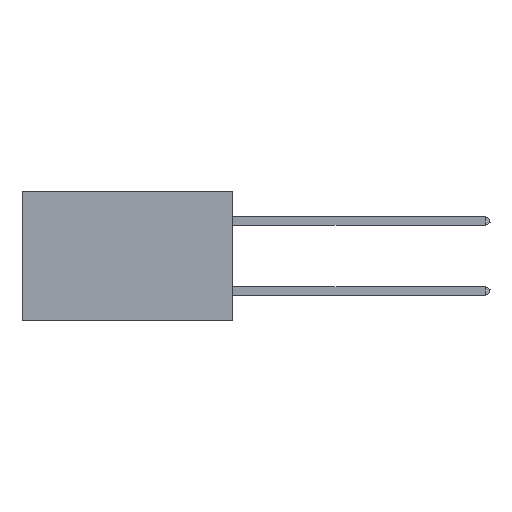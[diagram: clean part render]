
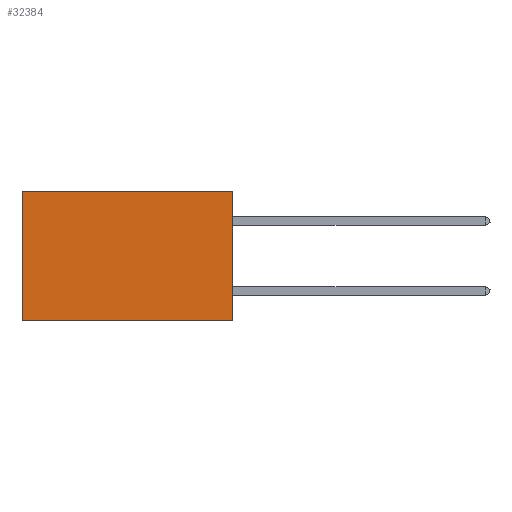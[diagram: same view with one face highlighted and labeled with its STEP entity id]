
A CAD part, left-side view. The second image highlights one B-rep face of the part: STEP entity #32384.
In plain terms, the highlighted planar face has unit normal (-1, 0, 0).
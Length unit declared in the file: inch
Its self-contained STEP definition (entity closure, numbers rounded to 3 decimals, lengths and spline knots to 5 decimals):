
#680 = EDGE_CURVE ( 'NONE', #29139, #26061, #40284, .T. ) ;
#997 = VECTOR ( 'NONE', #4630, 39.37008 ) ;
#1095 = ORIENTED_EDGE ( 'NONE', *, *, #31149, .T. ) ;
#1364 = CARTESIAN_POINT ( 'NONE',  ( 0.2875, 0., 0. ) ) ;
#2033 = DIRECTION ( 'NONE',  ( 0., 0., -1. ) ) ;
#3437 = LINE ( 'NONE', #18632, #30656 ) ;
#4630 = DIRECTION ( 'NONE',  ( 0., 1., 0. ) ) ;
#8059 = CARTESIAN_POINT ( 'NONE',  ( 0.2875, 0., 0. ) ) ;
#8118 = PLANE ( 'NONE',  #23854 ) ;
#8789 = CARTESIAN_POINT ( 'NONE',  ( 0.2875, 0.6, 0. ) ) ;
#10170 = CARTESIAN_POINT ( 'NONE',  ( 0.2875, 0., -0.37 ) ) ;
#10441 = VERTEX_POINT ( 'NONE', #27343 ) ;
#11585 = DIRECTION ( 'NONE',  ( 1., 0., 0. ) ) ;
#14887 = DIRECTION ( 'NONE',  ( 0., 1., 0. ) ) ;
#15821 = LINE ( 'NONE', #35925, #997 ) ;
#17450 = DIRECTION ( 'NONE',  ( 0., 0., -1. ) ) ;
#17477 = VECTOR ( 'NONE', #17450, 39.37008 ) ;
#18632 = CARTESIAN_POINT ( 'NONE',  ( 0.2875, 0.6, 0. ) ) ;
#20825 = CARTESIAN_POINT ( 'NONE',  ( 0.2875, 0., 0. ) ) ;
#23167 = LINE ( 'NONE', #37450, #35593 ) ;
#23475 = EDGE_CURVE ( 'NONE', #28111, #10441, #3437, .T. ) ;
#23854 = AXIS2_PLACEMENT_3D ( 'NONE', #20825, #11585, #2033 ) ;
#25884 = EDGE_LOOP ( 'NONE', ( #33829, #30295, #36092, #1095 ) ) ;
#26061 = VERTEX_POINT ( 'NONE', #10170 ) ;
#27343 = CARTESIAN_POINT ( 'NONE',  ( 0.2875, 0.6, -0.37 ) ) ;
#28111 = VERTEX_POINT ( 'NONE', #8789 ) ;
#29139 = VERTEX_POINT ( 'NONE', #1364 ) ;
#29758 = EDGE_CURVE ( 'NONE', #26061, #10441, #15821, .T. ) ;
#30295 = ORIENTED_EDGE ( 'NONE', *, *, #29758, .F. ) ;
#30656 = VECTOR ( 'NONE', #30829, 39.37008 ) ;
#30829 = DIRECTION ( 'NONE',  ( 0., 0., -1. ) ) ;
#31149 = EDGE_CURVE ( 'NONE', #29139, #28111, #23167, .T. ) ;
#32384 = ADVANCED_FACE ( 'NONE', ( #34502 ), #8118, .F. ) ;
#33829 = ORIENTED_EDGE ( 'NONE', *, *, #23475, .T. ) ;
#34502 = FACE_OUTER_BOUND ( 'NONE', #25884, .T. ) ;
#35593 = VECTOR ( 'NONE', #14887, 39.37008 ) ;
#35925 = CARTESIAN_POINT ( 'NONE',  ( 0.2875, 0., -0.37 ) ) ;
#36092 = ORIENTED_EDGE ( 'NONE', *, *, #680, .F. ) ;
#37450 = CARTESIAN_POINT ( 'NONE',  ( 0.2875, 0., 0. ) ) ;
#40284 = LINE ( 'NONE', #8059, #17477 ) ;
